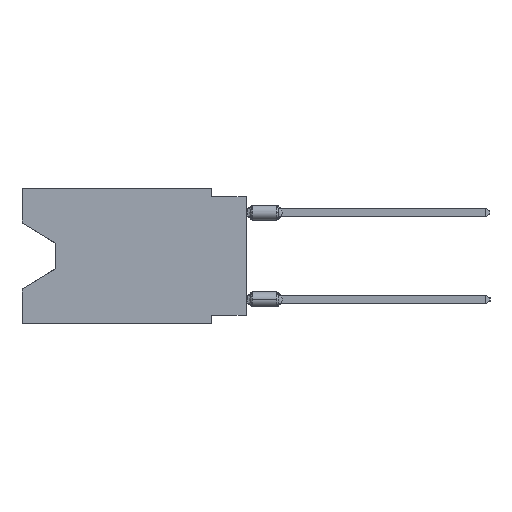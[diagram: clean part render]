
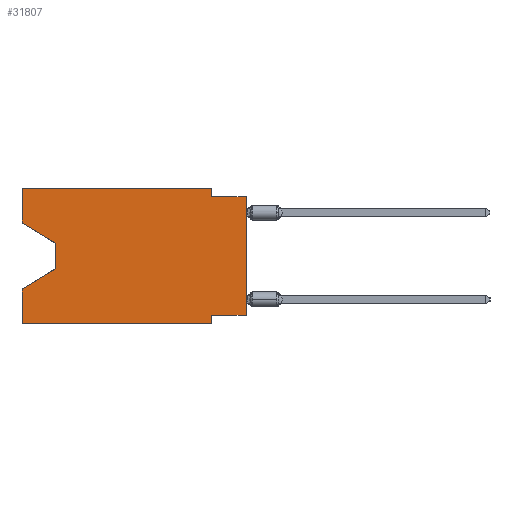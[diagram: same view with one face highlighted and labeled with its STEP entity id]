
A CAD part, left-side view. The second image highlights one B-rep face of the part: STEP entity #31807.
In plain terms, the highlighted planar face has unit normal (-1, 0, 0).
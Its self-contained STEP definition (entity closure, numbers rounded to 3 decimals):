
#8 = VECTOR ( 'NONE', #33119, 1000. ) ;
#142 = VERTEX_POINT ( 'NONE', #54417 ) ;
#271 = CARTESIAN_POINT ( 'NONE',  ( 0., 16.383, -7.36 ) ) ;
#528 = LINE ( 'NONE', #5240, #28681 ) ;
#1278 = ORIENTED_EDGE ( 'NONE', *, *, #21452, .T. ) ;
#1342 = VERTEX_POINT ( 'NONE', #50540 ) ;
#1422 = DIRECTION ( 'NONE',  ( 0., 0., -1. ) ) ;
#1839 = DIRECTION ( 'NONE',  ( 0., -1., 0. ) ) ;
#2115 = AXIS2_PLACEMENT_3D ( 'NONE', #9751, #6132, #1422 ) ;
#3690 = EDGE_CURVE ( 'NONE', #19603, #37903, #5037, .T. ) ;
#4150 = EDGE_CURVE ( 'NONE', #53691, #20328, #36602, .T. ) ;
#4326 = DIRECTION ( 'NONE',  ( 0., -0.855, -0.519 ) ) ;
#4724 = EDGE_CURVE ( 'NONE', #50649, #37903, #29163, .T. ) ;
#5037 = LINE ( 'NONE', #38157, #18730 ) ;
#5240 = CARTESIAN_POINT ( 'NONE',  ( 0., 0., -9.271 ) ) ;
#6132 = DIRECTION ( 'NONE',  ( 1., 0., 0. ) ) ;
#6713 = DIRECTION ( 'NONE',  ( 0., 0., -1. ) ) ;
#7145 = LINE ( 'NONE', #36660, #49812 ) ;
#7330 = EDGE_CURVE ( 'NONE', #50649, #25499, #528, .T. ) ;
#7842 = CARTESIAN_POINT ( 'NONE',  ( 0., 0., -0.635 ) ) ;
#7959 = DIRECTION ( 'NONE',  ( 0., 0., -1. ) ) ;
#9049 = CARTESIAN_POINT ( 'NONE',  ( 0., 13.97, -5.893 ) ) ;
#9751 = CARTESIAN_POINT ( 'NONE',  ( 0., 16.383, 0. ) ) ;
#11023 = ORIENTED_EDGE ( 'NONE', *, *, #4150, .F. ) ;
#11616 = CARTESIAN_POINT ( 'NONE',  ( 0., 0., -9.271 ) ) ;
#12928 = CARTESIAN_POINT ( 'NONE',  ( 0., 16.383, -2.546 ) ) ;
#13652 = LINE ( 'NONE', #31749, #8 ) ;
#14333 = EDGE_CURVE ( 'NONE', #53691, #35618, #22106, .T. ) ;
#14435 = EDGE_CURVE ( 'NONE', #1342, #25135, #30183, .T. ) ;
#14814 = VECTOR ( 'NONE', #6713, 1000. ) ;
#16757 = VECTOR ( 'NONE', #1839, 1000. ) ;
#18730 = VECTOR ( 'NONE', #52079, 1000. ) ;
#18819 = CARTESIAN_POINT ( 'NONE',  ( 0., 16.383, 0. ) ) ;
#19603 = VERTEX_POINT ( 'NONE', #48159 ) ;
#20034 = VERTEX_POINT ( 'NONE', #26264 ) ;
#20064 = DIRECTION ( 'NONE',  ( 0., -1., 0. ) ) ;
#20268 = DIRECTION ( 'NONE',  ( 0., 0., 1. ) ) ;
#20328 = VERTEX_POINT ( 'NONE', #50179 ) ;
#21438 = ORIENTED_EDGE ( 'NONE', *, *, #14435, .T. ) ;
#21452 = EDGE_CURVE ( 'NONE', #38340, #142, #27155, .T. ) ;
#22106 = LINE ( 'NONE', #12928, #30943 ) ;
#23395 = CARTESIAN_POINT ( 'NONE',  ( 0., 13.97, -4.013 ) ) ;
#23781 = DIRECTION ( 'NONE',  ( 0., 0., 1. ) ) ;
#24485 = CARTESIAN_POINT ( 'NONE',  ( 0., 16.383, -9.906 ) ) ;
#25135 = VERTEX_POINT ( 'NONE', #271 ) ;
#25300 = DIRECTION ( 'NONE',  ( 0., 0., 1. ) ) ;
#25396 = ORIENTED_EDGE ( 'NONE', *, *, #54736, .F. ) ;
#25499 = VERTEX_POINT ( 'NONE', #38543 ) ;
#26022 = DIRECTION ( 'NONE',  ( 0., 0.855, -0.519 ) ) ;
#26218 = EDGE_CURVE ( 'NONE', #20328, #20034, #28694, .T. ) ;
#26264 = CARTESIAN_POINT ( 'NONE',  ( 0., 2.54, 0. ) ) ;
#27103 = ORIENTED_EDGE ( 'NONE', *, *, #26218, .F. ) ;
#27155 = LINE ( 'NONE', #39958, #16757 ) ;
#28681 = VECTOR ( 'NONE', #42541, 1000. ) ;
#28694 = LINE ( 'NONE', #46214, #48227 ) ;
#29163 = LINE ( 'NONE', #50348, #48028 ) ;
#30183 = LINE ( 'NONE', #9049, #34525 ) ;
#30943 = VECTOR ( 'NONE', #4326, 1000. ) ;
#31459 = FACE_OUTER_BOUND ( 'NONE', #48942, .T. ) ;
#31749 = CARTESIAN_POINT ( 'NONE',  ( 0., 2.54, -9.906 ) ) ;
#31807 = ADVANCED_FACE ( 'NONE', ( #31459 ), #48458, .F. ) ;
#33119 = DIRECTION ( 'NONE',  ( 0., 0., -1. ) ) ;
#34525 = VECTOR ( 'NONE', #26022, 1000. ) ;
#34984 = EDGE_CURVE ( 'NONE', #35618, #1342, #45387, .T. ) ;
#35618 = VERTEX_POINT ( 'NONE', #51343 ) ;
#35977 = ORIENTED_EDGE ( 'NONE', *, *, #41167, .F. ) ;
#36602 = LINE ( 'NONE', #40758, #50664 ) ;
#36660 = CARTESIAN_POINT ( 'NONE',  ( 0., 2.54, 0. ) ) ;
#37903 = VERTEX_POINT ( 'NONE', #7842 ) ;
#38157 = CARTESIAN_POINT ( 'NONE',  ( 0., 0., -0.635 ) ) ;
#38340 = VERTEX_POINT ( 'NONE', #24485 ) ;
#38482 = EDGE_CURVE ( 'NONE', #38340, #25135, #42291, .T. ) ;
#38543 = CARTESIAN_POINT ( 'NONE',  ( 0., 2.54, -9.271 ) ) ;
#39565 = ORIENTED_EDGE ( 'NONE', *, *, #14333, .T. ) ;
#39958 = CARTESIAN_POINT ( 'NONE',  ( 0., 16.383, -9.906 ) ) ;
#40560 = ORIENTED_EDGE ( 'NONE', *, *, #3690, .F. ) ;
#40758 = CARTESIAN_POINT ( 'NONE',  ( 0., 16.383, 0. ) ) ;
#41167 = EDGE_CURVE ( 'NONE', #25499, #142, #13652, .T. ) ;
#41232 = ORIENTED_EDGE ( 'NONE', *, *, #34984, .T. ) ;
#41726 = VECTOR ( 'NONE', #25300, 1000. ) ;
#42291 = LINE ( 'NONE', #18819, #41726 ) ;
#42541 = DIRECTION ( 'NONE',  ( 0., 1., 0. ) ) ;
#43102 = ORIENTED_EDGE ( 'NONE', *, *, #38482, .F. ) ;
#44556 = ORIENTED_EDGE ( 'NONE', *, *, #7330, .F. ) ;
#45387 = LINE ( 'NONE', #23395, #14814 ) ;
#46214 = CARTESIAN_POINT ( 'NONE',  ( 0., 16.383, 0. ) ) ;
#48028 = VECTOR ( 'NONE', #20268, 1000. ) ;
#48159 = CARTESIAN_POINT ( 'NONE',  ( 0., 2.54, -0.635 ) ) ;
#48227 = VECTOR ( 'NONE', #20064, 1000. ) ;
#48458 = PLANE ( 'NONE',  #2115 ) ;
#48942 = EDGE_LOOP ( 'NONE', ( #39565, #41232, #21438, #43102, #1278, #35977, #44556, #53666, #40560, #25396, #27103, #11023 ) ) ;
#49812 = VECTOR ( 'NONE', #7959, 1000. ) ;
#50179 = CARTESIAN_POINT ( 'NONE',  ( 0., 16.383, 0. ) ) ;
#50348 = CARTESIAN_POINT ( 'NONE',  ( 0., 0., 0. ) ) ;
#50540 = CARTESIAN_POINT ( 'NONE',  ( 0., 13.97, -5.893 ) ) ;
#50649 = VERTEX_POINT ( 'NONE', #11616 ) ;
#50664 = VECTOR ( 'NONE', #23781, 1000. ) ;
#51093 = CARTESIAN_POINT ( 'NONE',  ( 0., 16.383, -2.546 ) ) ;
#51343 = CARTESIAN_POINT ( 'NONE',  ( 0., 13.97, -4.013 ) ) ;
#52079 = DIRECTION ( 'NONE',  ( 0., -1., 0. ) ) ;
#53666 = ORIENTED_EDGE ( 'NONE', *, *, #4724, .T. ) ;
#53691 = VERTEX_POINT ( 'NONE', #51093 ) ;
#54417 = CARTESIAN_POINT ( 'NONE',  ( 0., 2.54, -9.906 ) ) ;
#54736 = EDGE_CURVE ( 'NONE', #20034, #19603, #7145, .T. ) ;
